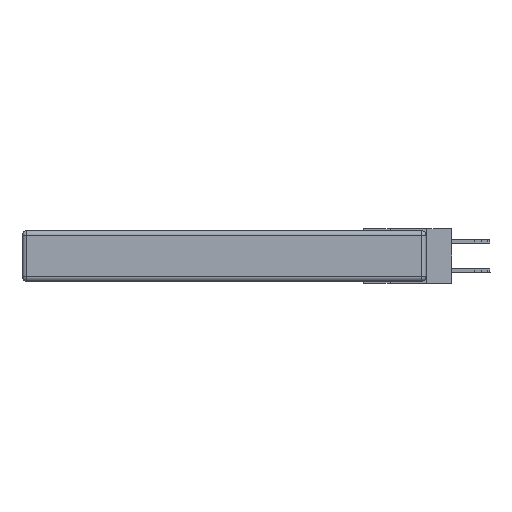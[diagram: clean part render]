
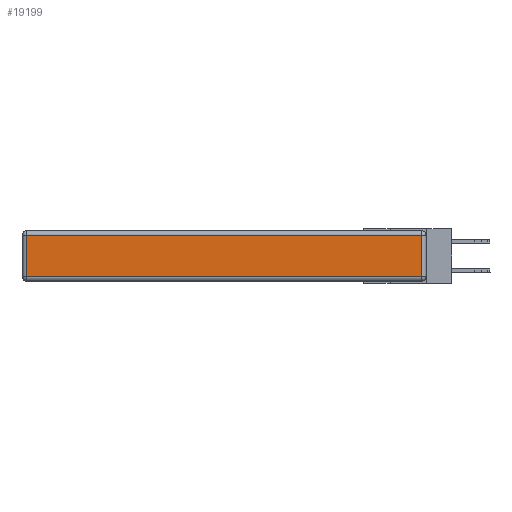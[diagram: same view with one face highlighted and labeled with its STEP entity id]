
A CAD part, left-side view. The second image highlights one B-rep face of the part: STEP entity #19199.
In plain terms, the highlighted planar face has unit normal (-1, 0, 0).
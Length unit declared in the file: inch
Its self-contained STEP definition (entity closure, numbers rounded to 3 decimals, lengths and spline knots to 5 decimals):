
#244 = VECTOR ( 'NONE', #10145, 39.37008 ) ;
#353 = EDGE_CURVE ( 'NONE', #7713, #14419, #10744, .T. ) ;
#1015 = CARTESIAN_POINT ( 'NONE',  ( 0., 2.75, -0.03 ) ) ;
#1651 = AXIS2_PLACEMENT_3D ( 'NONE', #14173, #18719, #8215 ) ;
#1792 = CARTESIAN_POINT ( 'NONE',  ( 0., 2.72, -0.343 ) ) ;
#2076 = LINE ( 'NONE', #11061, #6961 ) ;
#3214 = ORIENTED_EDGE ( 'NONE', *, *, #8690, .T. ) ;
#3590 = DIRECTION ( 'NONE',  ( 0., -1., 0. ) ) ;
#3902 = CARTESIAN_POINT ( 'NONE',  ( 0., 0.03, -0.343 ) ) ;
#4262 = DIRECTION ( 'NONE',  ( 0., 1., 0. ) ) ;
#5072 = ORIENTED_EDGE ( 'NONE', *, *, #353, .T. ) ;
#5149 = ORIENTED_EDGE ( 'NONE', *, *, #7030, .T. ) ;
#5349 = CARTESIAN_POINT ( 'NONE',  ( 0., 0.03, -0.313 ) ) ;
#5710 = ORIENTED_EDGE ( 'NONE', *, *, #12363, .T. ) ;
#6961 = VECTOR ( 'NONE', #3590, 39.37008 ) ;
#7030 = EDGE_CURVE ( 'NONE', #14419, #15410, #2076, .T. ) ;
#7644 = DIRECTION ( 'NONE',  ( 0., 0., -1. ) ) ;
#7704 = FACE_OUTER_BOUND ( 'NONE', #12600, .T. ) ;
#7713 = VERTEX_POINT ( 'NONE', #14819 ) ;
#8215 = DIRECTION ( 'NONE',  ( 0., 0., 1. ) ) ;
#8496 = VERTEX_POINT ( 'NONE', #12938 ) ;
#8690 = EDGE_CURVE ( 'NONE', #15410, #8496, #16792, .T. ) ;
#10023 = VECTOR ( 'NONE', #7644, 39.37008 ) ;
#10145 = DIRECTION ( 'NONE',  ( 0., 0., 1. ) ) ;
#10744 = LINE ( 'NONE', #1792, #10023 ) ;
#11061 = CARTESIAN_POINT ( 'NONE',  ( 0., 0., -0.313 ) ) ;
#11331 = PLANE ( 'NONE',  #1651 ) ;
#12363 = EDGE_CURVE ( 'NONE', #8496, #7713, #16125, .T. ) ;
#12600 = EDGE_LOOP ( 'NONE', ( #5149, #3214, #5710, #5072 ) ) ;
#12938 = CARTESIAN_POINT ( 'NONE',  ( 0., 0.03, -0.03 ) ) ;
#14173 = CARTESIAN_POINT ( 'NONE',  ( 0., 0., -0.343 ) ) ;
#14419 = VERTEX_POINT ( 'NONE', #15897 ) ;
#14819 = CARTESIAN_POINT ( 'NONE',  ( 0., 2.72, -0.03 ) ) ;
#15410 = VERTEX_POINT ( 'NONE', #5349 ) ;
#15448 = VECTOR ( 'NONE', #4262, 39.37008 ) ;
#15897 = CARTESIAN_POINT ( 'NONE',  ( 0., 2.72, -0.313 ) ) ;
#16125 = LINE ( 'NONE', #1015, #15448 ) ;
#16792 = LINE ( 'NONE', #3902, #244 ) ;
#18719 = DIRECTION ( 'NONE',  ( -1., 0., 0. ) ) ;
#19199 = ADVANCED_FACE ( 'NONE', ( #7704 ), #11331, .T. ) ;
